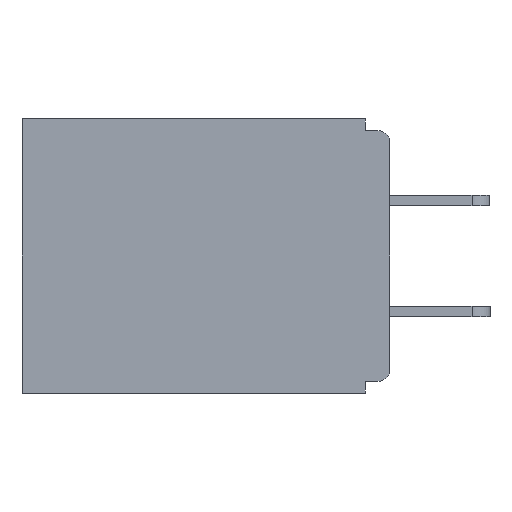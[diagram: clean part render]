
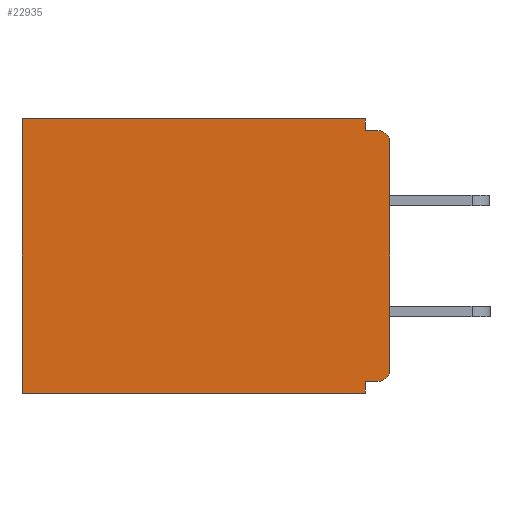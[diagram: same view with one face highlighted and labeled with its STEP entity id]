
A CAD part, left-side view. The second image highlights one B-rep face of the part: STEP entity #22935.
In plain terms, the highlighted planar face has unit normal (-1, 0, 0).
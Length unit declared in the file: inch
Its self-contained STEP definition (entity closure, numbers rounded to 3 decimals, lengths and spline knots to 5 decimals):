
#128 = ORIENTED_EDGE ( 'NONE', *, *, #6523, .T. ) ;
#213 = CARTESIAN_POINT ( 'NONE',  ( 0.298, 0.031, -0.015 ) ) ;
#220 = VERTEX_POINT ( 'NONE', #6340 ) ;
#334 = CARTESIAN_POINT ( 'NONE',  ( 0.298, 0., -0.03 ) ) ;
#732 = CIRCLE ( 'NONE', #19690, 0.015 ) ;
#1264 = VECTOR ( 'NONE', #2517, 39.37008 ) ;
#1342 = DIRECTION ( 'NONE',  ( 0., 1., 0. ) ) ;
#2517 = DIRECTION ( 'NONE',  ( 0., 0., -1. ) ) ;
#2520 = CARTESIAN_POINT ( 'NONE',  ( 0.298, 0.015, -0.328 ) ) ;
#2829 = CARTESIAN_POINT ( 'NONE',  ( 0.298, 0., -0.343 ) ) ;
#3194 = LINE ( 'NONE', #6757, #16517 ) ;
#3610 = DIRECTION ( 'NONE',  ( 0., 0., -1. ) ) ;
#3943 = EDGE_CURVE ( 'NONE', #8210, #11914, #6668, .T. ) ;
#4164 = VERTEX_POINT ( 'NONE', #15611 ) ;
#4367 = DIRECTION ( 'NONE',  ( -1., 0., 0. ) ) ;
#4517 = EDGE_CURVE ( 'NONE', #4164, #11829, #11469, .T. ) ;
#4810 = FACE_OUTER_BOUND ( 'NONE', #14200, .T. ) ;
#4920 = VERTEX_POINT ( 'NONE', #2520 ) ;
#5158 = EDGE_CURVE ( 'NONE', #4920, #9126, #732, .T. ) ;
#6340 = CARTESIAN_POINT ( 'NONE',  ( 0.298, 0.031, 0. ) ) ;
#6523 = EDGE_CURVE ( 'NONE', #15122, #11914, #12653, .T. ) ;
#6658 = EDGE_CURVE ( 'NONE', #220, #22192, #8148, .T. ) ;
#6668 = LINE ( 'NONE', #25142, #7623 ) ;
#6757 = CARTESIAN_POINT ( 'NONE',  ( 0.298, 0., 0. ) ) ;
#6819 = CARTESIAN_POINT ( 'NONE',  ( 0.298, 0.031, -0.343 ) ) ;
#7492 = LINE ( 'NONE', #18884, #8457 ) ;
#7573 = CARTESIAN_POINT ( 'NONE',  ( 0.298, 0., -0.313 ) ) ;
#7623 = VECTOR ( 'NONE', #16897, 39.37008 ) ;
#7638 = EDGE_CURVE ( 'NONE', #11829, #19706, #10992, .T. ) ;
#8148 = LINE ( 'NONE', #19888, #23992 ) ;
#8210 = VERTEX_POINT ( 'NONE', #213 ) ;
#8256 = CARTESIAN_POINT ( 'NONE',  ( 0.298, 0.46, -0.343 ) ) ;
#8457 = VECTOR ( 'NONE', #21067, 39.37008 ) ;
#9126 = VERTEX_POINT ( 'NONE', #7573 ) ;
#9313 = PLANE ( 'NONE',  #17889 ) ;
#10408 = ORIENTED_EDGE ( 'NONE', *, *, #4517, .F. ) ;
#10620 = CARTESIAN_POINT ( 'NONE',  ( 0.298, 0.46, 0. ) ) ;
#10662 = ORIENTED_EDGE ( 'NONE', *, *, #23450, .F. ) ;
#10992 = LINE ( 'NONE', #2829, #22674 ) ;
#11045 = CARTESIAN_POINT ( 'NONE',  ( 0.298, 0.031, -0.343 ) ) ;
#11244 = DIRECTION ( 'NONE',  ( 0., 1., 0. ) ) ;
#11332 = DIRECTION ( 'NONE',  ( 0., 1., 0. ) ) ;
#11469 = LINE ( 'NONE', #6819, #16346 ) ;
#11829 = VERTEX_POINT ( 'NONE', #11045 ) ;
#11914 = VERTEX_POINT ( 'NONE', #12851 ) ;
#12313 = ORIENTED_EDGE ( 'NONE', *, *, #15181, .T. ) ;
#12507 = ORIENTED_EDGE ( 'NONE', *, *, #5158, .T. ) ;
#12622 = DIRECTION ( 'NONE',  ( 0., 0., -1. ) ) ;
#12653 = CIRCLE ( 'NONE', #18162, 0.015 ) ;
#12851 = CARTESIAN_POINT ( 'NONE',  ( 0.298, 0.015, -0.015 ) ) ;
#14200 = EDGE_LOOP ( 'NONE', ( #128, #23478, #14659, #19497, #12313, #22906, #10408, #25817, #12507, #10662 ) ) ;
#14659 = ORIENTED_EDGE ( 'NONE', *, *, #22821, .F. ) ;
#14851 = DIRECTION ( 'NONE',  ( 0., 0., -1. ) ) ;
#15122 = VERTEX_POINT ( 'NONE', #334 ) ;
#15181 = EDGE_CURVE ( 'NONE', #22192, #19706, #7492, .T. ) ;
#15611 = CARTESIAN_POINT ( 'NONE',  ( 0.298, 0.031, -0.328 ) ) ;
#16346 = VECTOR ( 'NONE', #12622, 39.37008 ) ;
#16517 = VECTOR ( 'NONE', #25467, 39.37008 ) ;
#16897 = DIRECTION ( 'NONE',  ( 0., -1., 0. ) ) ;
#17169 = DIRECTION ( 'NONE',  ( 0., 0., -1. ) ) ;
#17889 = AXIS2_PLACEMENT_3D ( 'NONE', #23690, #25762, #17169 ) ;
#17895 = CARTESIAN_POINT ( 'NONE',  ( 0.298, 0.015, -0.313 ) ) ;
#18162 = AXIS2_PLACEMENT_3D ( 'NONE', #24995, #4367, #14851 ) ;
#18884 = CARTESIAN_POINT ( 'NONE',  ( 0.298, 0.46, 0. ) ) ;
#18895 = VECTOR ( 'NONE', #11332, 39.37008 ) ;
#19497 = ORIENTED_EDGE ( 'NONE', *, *, #6658, .T. ) ;
#19690 = AXIS2_PLACEMENT_3D ( 'NONE', #17895, #24067, #3610 ) ;
#19706 = VERTEX_POINT ( 'NONE', #8256 ) ;
#19888 = CARTESIAN_POINT ( 'NONE',  ( 0.298, 0., 0. ) ) ;
#20224 = LINE ( 'NONE', #21927, #18895 ) ;
#20460 = EDGE_CURVE ( 'NONE', #4920, #4164, #20224, .T. ) ;
#20718 = LINE ( 'NONE', #23178, #1264 ) ;
#21067 = DIRECTION ( 'NONE',  ( 0., 0., -1. ) ) ;
#21927 = CARTESIAN_POINT ( 'NONE',  ( 0.298, 0., -0.328 ) ) ;
#22192 = VERTEX_POINT ( 'NONE', #10620 ) ;
#22674 = VECTOR ( 'NONE', #11244, 39.37008 ) ;
#22821 = EDGE_CURVE ( 'NONE', #220, #8210, #20718, .T. ) ;
#22906 = ORIENTED_EDGE ( 'NONE', *, *, #7638, .F. ) ;
#22935 = ADVANCED_FACE ( 'NONE', ( #4810 ), #9313, .F. ) ;
#23178 = CARTESIAN_POINT ( 'NONE',  ( 0.298, 0.031, -0.343 ) ) ;
#23450 = EDGE_CURVE ( 'NONE', #15122, #9126, #3194, .T. ) ;
#23478 = ORIENTED_EDGE ( 'NONE', *, *, #3943, .F. ) ;
#23690 = CARTESIAN_POINT ( 'NONE',  ( 0.298, 0., 0. ) ) ;
#23992 = VECTOR ( 'NONE', #1342, 39.37008 ) ;
#24067 = DIRECTION ( 'NONE',  ( -1., 0., 0. ) ) ;
#24995 = CARTESIAN_POINT ( 'NONE',  ( 0.298, 0.015, -0.03 ) ) ;
#25142 = CARTESIAN_POINT ( 'NONE',  ( 0.298, 0., -0.015 ) ) ;
#25467 = DIRECTION ( 'NONE',  ( 0., 0., -1. ) ) ;
#25762 = DIRECTION ( 'NONE',  ( 1., 0., 0. ) ) ;
#25817 = ORIENTED_EDGE ( 'NONE', *, *, #20460, .F. ) ;
